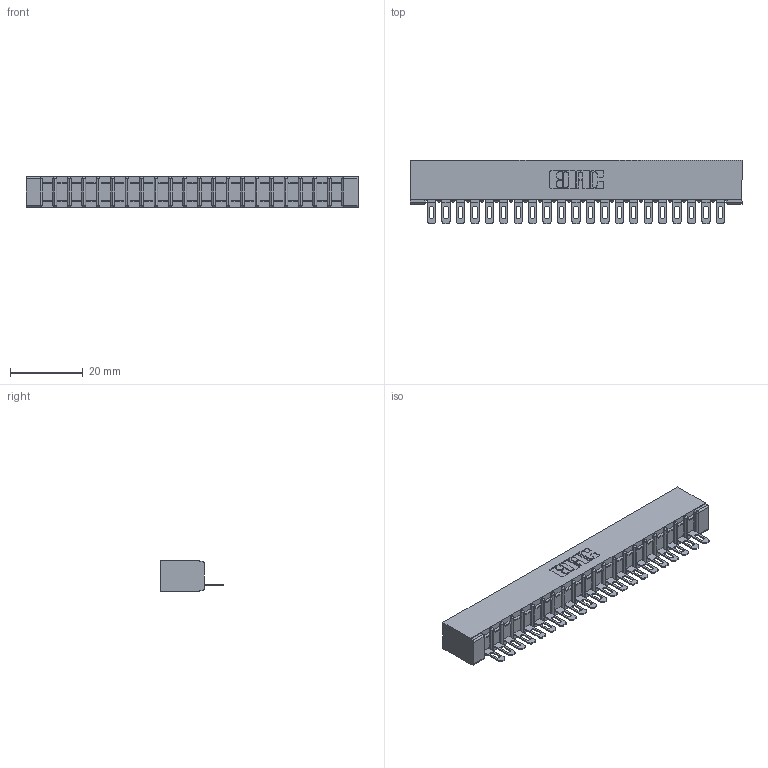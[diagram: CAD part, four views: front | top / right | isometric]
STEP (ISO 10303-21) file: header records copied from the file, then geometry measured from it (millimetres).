
FILE_DESCRIPTION (( 'STEP AP203' ), '1' );
FILE_NAME ('357-021-401-101.STEP', '2020-10-01T06:19:21', ( '' ), ( '' ), 'SwSTEP 2.0', 'SolidWorks 2020', '' );
FILE_SCHEMA (( 'CONFIG_CONTROL_DESIGN' ));
Length unit declared in the file: inch
Products named in the file (3): 307 Part_No Mounting Lugs; 307-290-002_501; 357-021-401-101
Assembly tree (22 placements, depth 2):
  357-021-401-101
    307 Part_No Mounting Lugs
    307-290-002_501  x21
Bounding box: 91.08 x 17.42 x 8.71 mm (x, y, z)
Volume: 6273.3 mm3; surface area: 12003 mm2
Topology: 22 solids, 22 shells, 1728 faces, 5297 edges, 3470 vertices
Faces by surface type: plane 990, cylinder 694, sphere 44
Entity records: 21108 total; most frequent: CARTESIAN_POINT 3556, ORIENTED_EDGE 3546, DIRECTION 3467, EDGE_CURVE 1773, LINE 1345, VECTOR 1345, VERTEX_POINT 1150, AXIS2_PLACEMENT_3D 1061
